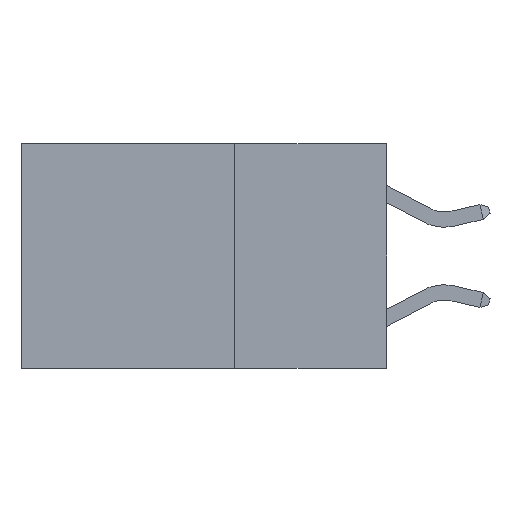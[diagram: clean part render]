
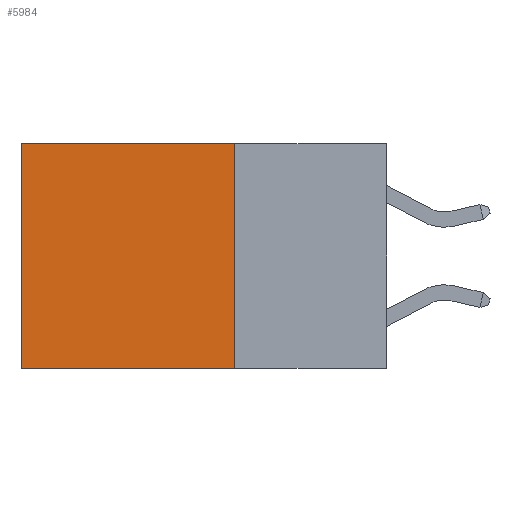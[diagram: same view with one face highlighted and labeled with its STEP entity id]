
A CAD part, left-side view. The second image highlights one B-rep face of the part: STEP entity #5984.
In plain terms, the highlighted planar face has unit normal (-1, 0, 0).
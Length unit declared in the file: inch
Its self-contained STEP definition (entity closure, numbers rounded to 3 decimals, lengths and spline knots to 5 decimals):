
#327 = AXIS2_PLACEMENT_3D ( 'NONE', #12854, #12636, #4283 ) ;
#377 = LINE ( 'NONE', #3509, #7594 ) ;
#946 = DIRECTION ( 'NONE',  ( 0., 1., 0. ) ) ;
#1082 = FACE_OUTER_BOUND ( 'NONE', #20377, .T. ) ;
#1095 = CARTESIAN_POINT ( 'NONE',  ( 0.2625, 0.6, -0.37 ) ) ;
#1399 = VECTOR ( 'NONE', #946, 39.37008 ) ;
#2146 = VERTEX_POINT ( 'NONE', #4551 ) ;
#2963 = DIRECTION ( 'NONE',  ( 0., 0., -1. ) ) ;
#3509 = CARTESIAN_POINT ( 'NONE',  ( 0.2625, 0.6, 0. ) ) ;
#4028 = CARTESIAN_POINT ( 'NONE',  ( 0.2625, 0.25, -0.37 ) ) ;
#4137 = ORIENTED_EDGE ( 'NONE', *, *, #10884, .T. ) ;
#4283 = DIRECTION ( 'NONE',  ( 0., 0., -1. ) ) ;
#4551 = CARTESIAN_POINT ( 'NONE',  ( 0.2625, 0.25, -0.37 ) ) ;
#4730 = CARTESIAN_POINT ( 'NONE',  ( 0.2625, 0.25, 0. ) ) ;
#5364 = LINE ( 'NONE', #12168, #10428 ) ;
#5984 = ADVANCED_FACE ( 'NONE', ( #1082 ), #17650, .F. ) ;
#6814 = ORIENTED_EDGE ( 'NONE', *, *, #20730, .T. ) ;
#7594 = VECTOR ( 'NONE', #10179, 39.37008 ) ;
#10179 = DIRECTION ( 'NONE',  ( 0., 0., -1. ) ) ;
#10428 = VECTOR ( 'NONE', #18964, 39.37008 ) ;
#10822 = ORIENTED_EDGE ( 'NONE', *, *, #18299, .F. ) ;
#10884 = EDGE_CURVE ( 'NONE', #11705, #11980, #377, .T. ) ;
#11182 = VECTOR ( 'NONE', #2963, 39.37008 ) ;
#11705 = VERTEX_POINT ( 'NONE', #21680 ) ;
#11980 = VERTEX_POINT ( 'NONE', #1095 ) ;
#12075 = EDGE_CURVE ( 'NONE', #12135, #2146, #14761, .T. ) ;
#12135 = VERTEX_POINT ( 'NONE', #4730 ) ;
#12168 = CARTESIAN_POINT ( 'NONE',  ( 0.2625, 0.25, 0. ) ) ;
#12636 = DIRECTION ( 'NONE',  ( 1., 0., 0. ) ) ;
#12854 = CARTESIAN_POINT ( 'NONE',  ( 0.2625, 0.25, 0. ) ) ;
#14510 = LINE ( 'NONE', #4028, #1399 ) ;
#14761 = LINE ( 'NONE', #15202, #11182 ) ;
#15202 = CARTESIAN_POINT ( 'NONE',  ( 0.2625, 0.25, 0. ) ) ;
#15500 = ORIENTED_EDGE ( 'NONE', *, *, #12075, .F. ) ;
#17650 = PLANE ( 'NONE',  #327 ) ;
#18299 = EDGE_CURVE ( 'NONE', #2146, #11980, #14510, .T. ) ;
#18964 = DIRECTION ( 'NONE',  ( 0., 1., 0. ) ) ;
#20377 = EDGE_LOOP ( 'NONE', ( #4137, #10822, #15500, #6814 ) ) ;
#20730 = EDGE_CURVE ( 'NONE', #12135, #11705, #5364, .T. ) ;
#21680 = CARTESIAN_POINT ( 'NONE',  ( 0.2625, 0.6, 0. ) ) ;
